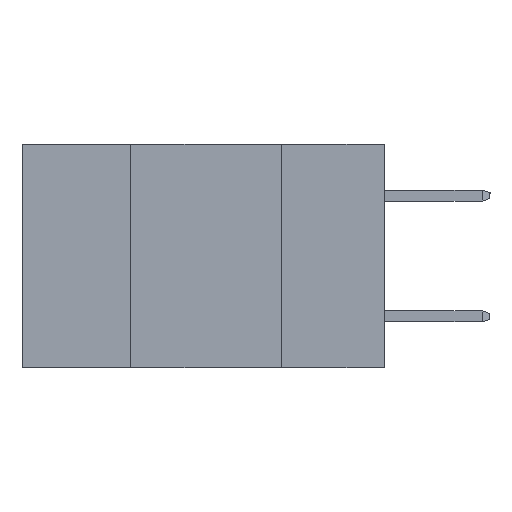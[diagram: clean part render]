
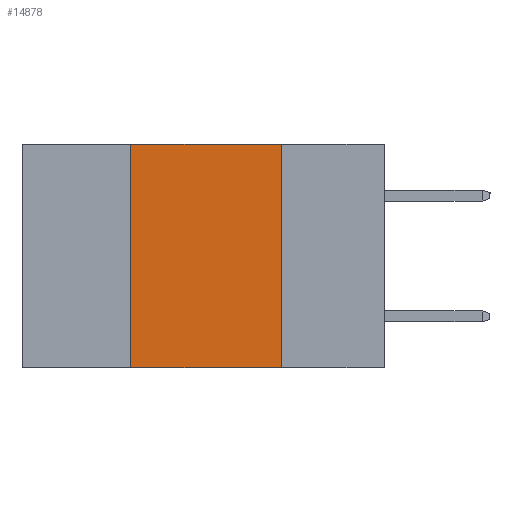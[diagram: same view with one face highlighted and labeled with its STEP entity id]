
A CAD part, left-side view. The second image highlights one B-rep face of the part: STEP entity #14878.
In plain terms, the highlighted planar face has unit normal (-1, 0, 0).
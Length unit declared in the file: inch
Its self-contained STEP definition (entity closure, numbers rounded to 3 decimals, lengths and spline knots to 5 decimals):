
#181 = CARTESIAN_POINT ( 'NONE',  ( 0., 0.42, -0.37 ) ) ;
#316 = DIRECTION ( 'NONE',  ( 0., 0., -1. ) ) ;
#390 = PLANE ( 'NONE',  #4972 ) ;
#494 = CARTESIAN_POINT ( 'NONE',  ( 0., 0.17, 0. ) ) ;
#953 = EDGE_CURVE ( 'NONE', #13749, #12983, #5260, .T. ) ;
#1366 = ORIENTED_EDGE ( 'NONE', *, *, #15472, .F. ) ;
#1767 = LINE ( 'NONE', #7911, #14919 ) ;
#2206 = ORIENTED_EDGE ( 'NONE', *, *, #12523, .F. ) ;
#2468 = VERTEX_POINT ( 'NONE', #14486 ) ;
#2803 = LINE ( 'NONE', #7586, #8464 ) ;
#2808 = CARTESIAN_POINT ( 'NONE',  ( 0., 0.17, -0.37 ) ) ;
#3933 = VECTOR ( 'NONE', #10460, 39.37008 ) ;
#4483 = EDGE_CURVE ( 'NONE', #12817, #12983, #11654, .T. ) ;
#4972 = AXIS2_PLACEMENT_3D ( 'NONE', #10008, #14832, #316 ) ;
#5260 = LINE ( 'NONE', #2808, #10729 ) ;
#6720 = ORIENTED_EDGE ( 'NONE', *, *, #4483, .T. ) ;
#7586 = CARTESIAN_POINT ( 'NONE',  ( 0., 0.42, -0.37 ) ) ;
#7828 = DIRECTION ( 'NONE',  ( 0., -1., 0. ) ) ;
#7889 = CARTESIAN_POINT ( 'NONE',  ( 0., 0.17, -0.37 ) ) ;
#7911 = CARTESIAN_POINT ( 'NONE',  ( 0., 0.6, 0. ) ) ;
#8027 = ORIENTED_EDGE ( 'NONE', *, *, #953, .F. ) ;
#8464 = VECTOR ( 'NONE', #12416, 39.37008 ) ;
#10008 = CARTESIAN_POINT ( 'NONE',  ( 0., 0.6, 0. ) ) ;
#10049 = DIRECTION ( 'NONE',  ( 0., 0., -1. ) ) ;
#10460 = DIRECTION ( 'NONE',  ( 0., -1., 0. ) ) ;
#10729 = VECTOR ( 'NONE', #10049, 39.37008 ) ;
#11183 = FACE_OUTER_BOUND ( 'NONE', #11227, .T. ) ;
#11227 = EDGE_LOOP ( 'NONE', ( #8027, #2206, #1366, #6720 ) ) ;
#11654 = LINE ( 'NONE', #13052, #3933 ) ;
#12416 = DIRECTION ( 'NONE',  ( 0., 0., 1. ) ) ;
#12523 = EDGE_CURVE ( 'NONE', #2468, #13749, #1767, .T. ) ;
#12817 = VERTEX_POINT ( 'NONE', #181 ) ;
#12983 = VERTEX_POINT ( 'NONE', #7889 ) ;
#13052 = CARTESIAN_POINT ( 'NONE',  ( 0., 0.6, -0.37 ) ) ;
#13749 = VERTEX_POINT ( 'NONE', #494 ) ;
#14486 = CARTESIAN_POINT ( 'NONE',  ( 0., 0.42, 0. ) ) ;
#14832 = DIRECTION ( 'NONE',  ( 1., 0., 0. ) ) ;
#14878 = ADVANCED_FACE ( 'NONE', ( #11183 ), #390, .F. ) ;
#14919 = VECTOR ( 'NONE', #7828, 39.37008 ) ;
#15472 = EDGE_CURVE ( 'NONE', #12817, #2468, #2803, .T. ) ;
